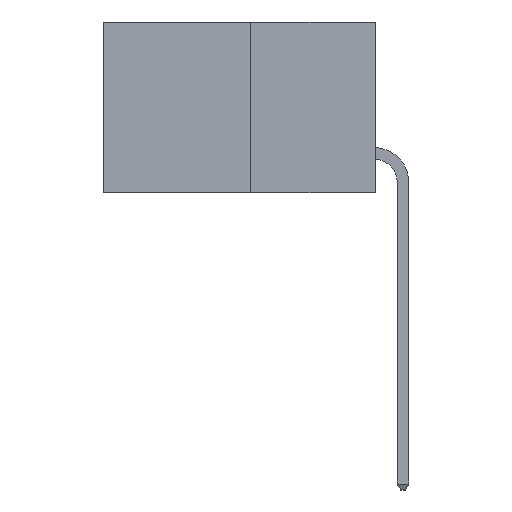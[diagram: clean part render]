
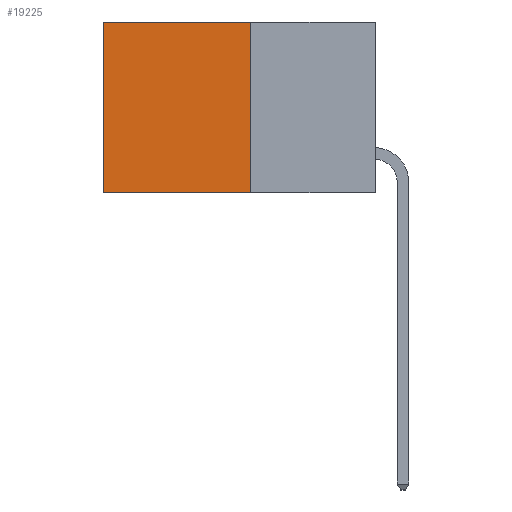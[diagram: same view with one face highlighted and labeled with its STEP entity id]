
A CAD part, left-side view. The second image highlights one B-rep face of the part: STEP entity #19225.
In plain terms, the highlighted planar face has unit normal (-1, 0, 0).
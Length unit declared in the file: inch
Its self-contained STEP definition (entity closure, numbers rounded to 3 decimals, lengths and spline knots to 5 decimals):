
#1136 = ORIENTED_EDGE ( 'NONE', *, *, #4620, .T. ) ;
#1175 = VECTOR ( 'NONE', #5878, 39.37008 ) ;
#1554 = CARTESIAN_POINT ( 'NONE',  ( 0.277, 0.27, 0. ) ) ;
#1829 = EDGE_LOOP ( 'NONE', ( #1136, #3277, #20478, #8946 ) ) ;
#3277 = ORIENTED_EDGE ( 'NONE', *, *, #14046, .F. ) ;
#3824 = LINE ( 'NONE', #16123, #8216 ) ;
#4089 = LINE ( 'NONE', #5564, #7960 ) ;
#4620 = EDGE_CURVE ( 'NONE', #6234, #20284, #3824, .T. ) ;
#5525 = LINE ( 'NONE', #12344, #1175 ) ;
#5564 = CARTESIAN_POINT ( 'NONE',  ( 0.277, 0.27, 0. ) ) ;
#5605 = CARTESIAN_POINT ( 'NONE',  ( 0.277, 0.59, 0. ) ) ;
#5617 = AXIS2_PLACEMENT_3D ( 'NONE', #9001, #20263, #10631 ) ;
#5878 = DIRECTION ( 'NONE',  ( 0., 0., -1. ) ) ;
#6234 = VERTEX_POINT ( 'NONE', #5605 ) ;
#6742 = CARTESIAN_POINT ( 'NONE',  ( 0.277, 0.59, -0.37 ) ) ;
#7312 = DIRECTION ( 'NONE',  ( 0., 1., 0. ) ) ;
#7360 = PLANE ( 'NONE',  #5617 ) ;
#7671 = CARTESIAN_POINT ( 'NONE',  ( 0.277, 0.27, -0.37 ) ) ;
#7960 = VECTOR ( 'NONE', #7312, 39.37008 ) ;
#8216 = VECTOR ( 'NONE', #11239, 39.37008 ) ;
#8543 = FACE_OUTER_BOUND ( 'NONE', #1829, .T. ) ;
#8946 = ORIENTED_EDGE ( 'NONE', *, *, #20467, .T. ) ;
#9001 = CARTESIAN_POINT ( 'NONE',  ( 0.277, 0.27, -0.37 ) ) ;
#9293 = VERTEX_POINT ( 'NONE', #1554 ) ;
#10631 = DIRECTION ( 'NONE',  ( 0., 0., -1. ) ) ;
#10828 = CARTESIAN_POINT ( 'NONE',  ( 0.277, 0.27, -0.37 ) ) ;
#11239 = DIRECTION ( 'NONE',  ( 0., 0., -1. ) ) ;
#11244 = LINE ( 'NONE', #10828, #15054 ) ;
#12344 = CARTESIAN_POINT ( 'NONE',  ( 0.277, 0.27, -0.37 ) ) ;
#14046 = EDGE_CURVE ( 'NONE', #16022, #20284, #11244, .T. ) ;
#15054 = VECTOR ( 'NONE', #18876, 39.37008 ) ;
#16022 = VERTEX_POINT ( 'NONE', #7671 ) ;
#16123 = CARTESIAN_POINT ( 'NONE',  ( 0.277, 0.59, -0.37 ) ) ;
#17271 = EDGE_CURVE ( 'NONE', #9293, #16022, #5525, .T. ) ;
#18876 = DIRECTION ( 'NONE',  ( 0., 1., 0. ) ) ;
#19225 = ADVANCED_FACE ( 'NONE', ( #8543 ), #7360, .F. ) ;
#20263 = DIRECTION ( 'NONE',  ( 1., 0., 0. ) ) ;
#20284 = VERTEX_POINT ( 'NONE', #6742 ) ;
#20467 = EDGE_CURVE ( 'NONE', #9293, #6234, #4089, .T. ) ;
#20478 = ORIENTED_EDGE ( 'NONE', *, *, #17271, .F. ) ;
